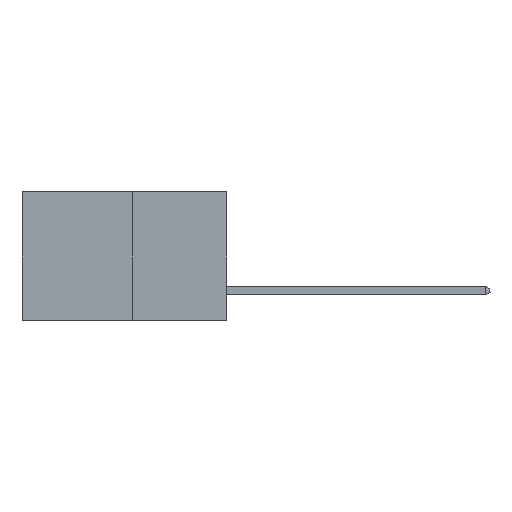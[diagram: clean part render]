
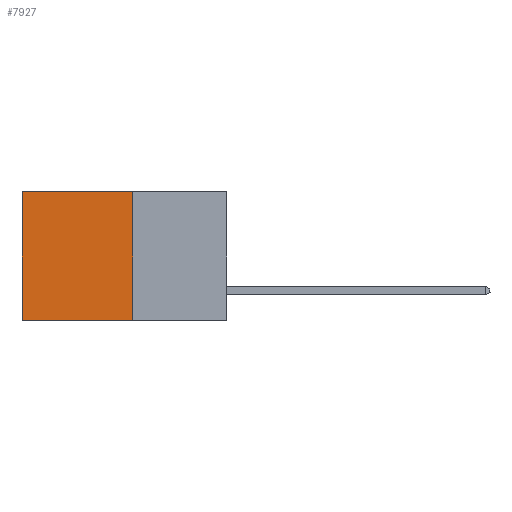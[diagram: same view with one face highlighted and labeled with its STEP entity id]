
A CAD part, left-side view. The second image highlights one B-rep face of the part: STEP entity #7927.
In plain terms, the highlighted planar face has unit normal (-1, 0, 0).
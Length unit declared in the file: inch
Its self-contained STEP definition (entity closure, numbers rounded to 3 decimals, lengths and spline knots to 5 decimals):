
#594 = VERTEX_POINT ( 'NONE', #5774 ) ;
#665 = AXIS2_PLACEMENT_3D ( 'NONE', #1825, #7083, #2591 ) ;
#772 = LINE ( 'NONE', #2677, #8265 ) ;
#1076 = VECTOR ( 'NONE', #8924, 39.37008 ) ;
#1338 = ORIENTED_EDGE ( 'NONE', *, *, #3186, .T. ) ;
#1653 = DIRECTION ( 'NONE',  ( 0., 1., 0. ) ) ;
#1825 = CARTESIAN_POINT ( 'NONE',  ( 0.277, 0.27, -0.37 ) ) ;
#1830 = VERTEX_POINT ( 'NONE', #6941 ) ;
#1838 = ORIENTED_EDGE ( 'NONE', *, *, #7837, .T. ) ;
#2189 = VERTEX_POINT ( 'NONE', #7257 ) ;
#2241 = LINE ( 'NONE', #6934, #8349 ) ;
#2360 = VECTOR ( 'NONE', #8157, 39.37008 ) ;
#2579 = CARTESIAN_POINT ( 'NONE',  ( 0.277, 0.27, 0. ) ) ;
#2591 = DIRECTION ( 'NONE',  ( 0., 0., -1. ) ) ;
#2677 = CARTESIAN_POINT ( 'NONE',  ( 0.277, 0.27, -0.37 ) ) ;
#3186 = EDGE_CURVE ( 'NONE', #1830, #594, #4406, .T. ) ;
#3822 = CARTESIAN_POINT ( 'NONE',  ( 0.277, 0.27, -0.37 ) ) ;
#4406 = LINE ( 'NONE', #5558, #2360 ) ;
#5558 = CARTESIAN_POINT ( 'NONE',  ( 0.277, 0.59, -0.37 ) ) ;
#5753 = DIRECTION ( 'NONE',  ( 0., 0., -1. ) ) ;
#5774 = CARTESIAN_POINT ( 'NONE',  ( 0.277, 0.59, -0.37 ) ) ;
#6134 = EDGE_CURVE ( 'NONE', #7065, #2189, #772, .T. ) ;
#6363 = PLANE ( 'NONE',  #665 ) ;
#6897 = LINE ( 'NONE', #3822, #1076 ) ;
#6934 = CARTESIAN_POINT ( 'NONE',  ( 0.277, 0.27, 0. ) ) ;
#6941 = CARTESIAN_POINT ( 'NONE',  ( 0.277, 0.59, 0. ) ) ;
#7065 = VERTEX_POINT ( 'NONE', #2579 ) ;
#7083 = DIRECTION ( 'NONE',  ( 1., 0., 0. ) ) ;
#7257 = CARTESIAN_POINT ( 'NONE',  ( 0.277, 0.27, -0.37 ) ) ;
#7327 = EDGE_LOOP ( 'NONE', ( #1338, #7577, #7368, #1838 ) ) ;
#7368 = ORIENTED_EDGE ( 'NONE', *, *, #6134, .F. ) ;
#7577 = ORIENTED_EDGE ( 'NONE', *, *, #9462, .F. ) ;
#7837 = EDGE_CURVE ( 'NONE', #7065, #1830, #2241, .T. ) ;
#7927 = ADVANCED_FACE ( 'NONE', ( #8245 ), #6363, .F. ) ;
#8157 = DIRECTION ( 'NONE',  ( 0., 0., -1. ) ) ;
#8245 = FACE_OUTER_BOUND ( 'NONE', #7327, .T. ) ;
#8265 = VECTOR ( 'NONE', #5753, 39.37008 ) ;
#8349 = VECTOR ( 'NONE', #1653, 39.37008 ) ;
#8924 = DIRECTION ( 'NONE',  ( 0., 1., 0. ) ) ;
#9462 = EDGE_CURVE ( 'NONE', #2189, #594, #6897, .T. ) ;
